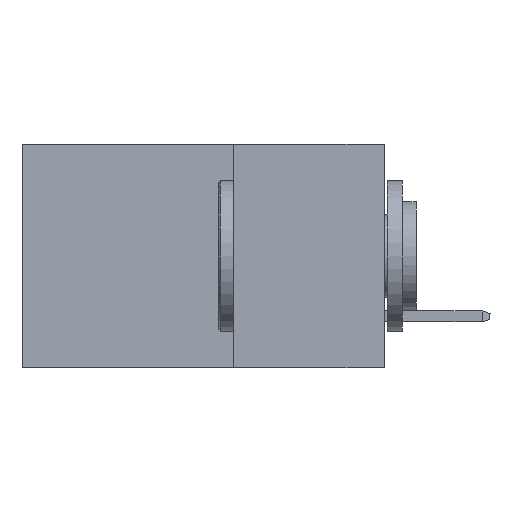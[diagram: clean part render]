
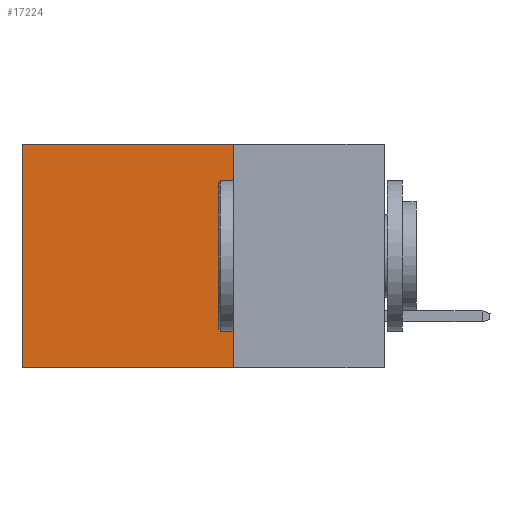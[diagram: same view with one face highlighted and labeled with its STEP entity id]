
A CAD part, left-side view. The second image highlights one B-rep face of the part: STEP entity #17224.
In plain terms, the highlighted planar face has unit normal (-1, 0, 0).
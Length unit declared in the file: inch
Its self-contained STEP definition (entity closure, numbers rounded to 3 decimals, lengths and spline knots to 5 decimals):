
#621 = CARTESIAN_POINT ( 'NONE',  ( 0.2615, 0.25, 0. ) ) ;
#1637 = EDGE_CURVE ( 'NONE', #22415, #14169, #4274, .T. ) ;
#2558 = EDGE_CURVE ( 'NONE', #21436, #22415, #11354, .T. ) ;
#2627 = VERTEX_POINT ( 'NONE', #20701 ) ;
#4274 = LINE ( 'NONE', #7650, #13681 ) ;
#4511 = DIRECTION ( 'NONE',  ( 0., 0., -1. ) ) ;
#4684 = ORIENTED_EDGE ( 'NONE', *, *, #1637, .T. ) ;
#4722 = CARTESIAN_POINT ( 'NONE',  ( 0.2615, 0.25, -0.37 ) ) ;
#4849 = LINE ( 'NONE', #4722, #23590 ) ;
#5032 = CARTESIAN_POINT ( 'NONE',  ( 0.2615, 0.25, -0.37 ) ) ;
#5600 = EDGE_LOOP ( 'NONE', ( #4684, #11662, #13338, #14550 ) ) ;
#6589 = FACE_OUTER_BOUND ( 'NONE', #5600, .T. ) ;
#7371 = CARTESIAN_POINT ( 'NONE',  ( 0.2615, 0.25, 0. ) ) ;
#7650 = CARTESIAN_POINT ( 'NONE',  ( 0.2615, 0.6, -0.37 ) ) ;
#7965 = VECTOR ( 'NONE', #14601, 39.37008 ) ;
#11242 = DIRECTION ( 'NONE',  ( 0., 1., 0. ) ) ;
#11354 = LINE ( 'NONE', #7371, #22651 ) ;
#11662 = ORIENTED_EDGE ( 'NONE', *, *, #18950, .F. ) ;
#11905 = CARTESIAN_POINT ( 'NONE',  ( 0.2615, 0.25, -0.37 ) ) ;
#12445 = CARTESIAN_POINT ( 'NONE',  ( 0.2615, 0.6, 0. ) ) ;
#13338 = ORIENTED_EDGE ( 'NONE', *, *, #15770, .F. ) ;
#13681 = VECTOR ( 'NONE', #17127, 39.37008 ) ;
#13715 = DIRECTION ( 'NONE',  ( 1., 0., 0. ) ) ;
#14169 = VERTEX_POINT ( 'NONE', #23736 ) ;
#14550 = ORIENTED_EDGE ( 'NONE', *, *, #2558, .T. ) ;
#14601 = DIRECTION ( 'NONE',  ( 0., 0., -1. ) ) ;
#14622 = AXIS2_PLACEMENT_3D ( 'NONE', #11905, #13715, #4511 ) ;
#15770 = EDGE_CURVE ( 'NONE', #21436, #2627, #20304, .T. ) ;
#17127 = DIRECTION ( 'NONE',  ( 0., 0., -1. ) ) ;
#17224 = ADVANCED_FACE ( 'NONE', ( #6589 ), #19550, .F. ) ;
#18950 = EDGE_CURVE ( 'NONE', #2627, #14169, #4849, .T. ) ;
#19286 = DIRECTION ( 'NONE',  ( 0., 1., 0. ) ) ;
#19550 = PLANE ( 'NONE',  #14622 ) ;
#20304 = LINE ( 'NONE', #5032, #7965 ) ;
#20701 = CARTESIAN_POINT ( 'NONE',  ( 0.2615, 0.25, -0.37 ) ) ;
#21436 = VERTEX_POINT ( 'NONE', #621 ) ;
#22415 = VERTEX_POINT ( 'NONE', #12445 ) ;
#22651 = VECTOR ( 'NONE', #11242, 39.37008 ) ;
#23590 = VECTOR ( 'NONE', #19286, 39.37008 ) ;
#23736 = CARTESIAN_POINT ( 'NONE',  ( 0.2615, 0.6, -0.37 ) ) ;
